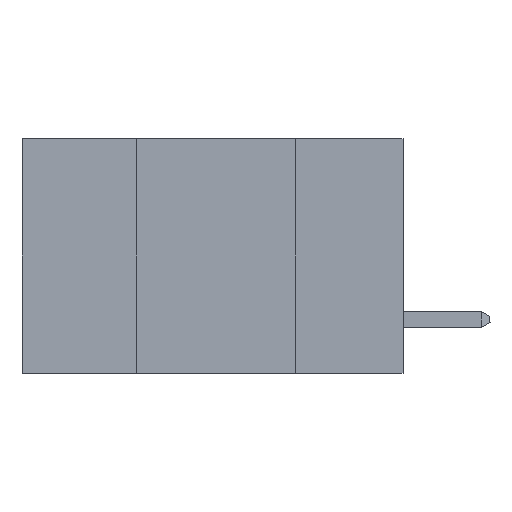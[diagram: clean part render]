
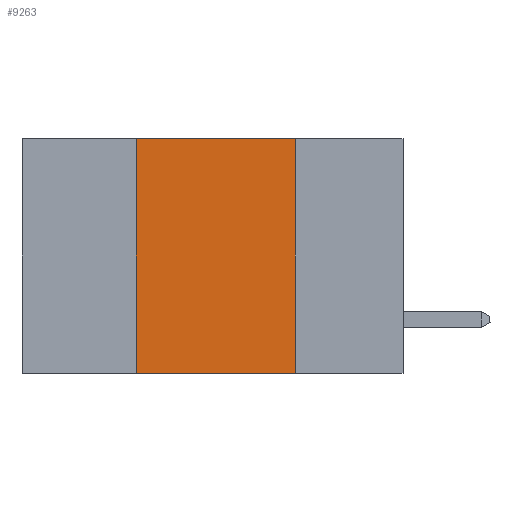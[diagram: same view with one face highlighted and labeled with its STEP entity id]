
A CAD part, left-side view. The second image highlights one B-rep face of the part: STEP entity #9263.
In plain terms, the highlighted planar face has unit normal (-1, 0, 0).
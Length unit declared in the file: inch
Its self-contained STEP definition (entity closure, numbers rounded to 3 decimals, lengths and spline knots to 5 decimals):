
#271 = CARTESIAN_POINT ( 'NONE',  ( 0., 0.6, 0. ) ) ;
#1824 = LINE ( 'NONE', #16335, #13165 ) ;
#4355 = VECTOR ( 'NONE', #14549, 39.37008 ) ;
#4760 = LINE ( 'NONE', #27559, #16158 ) ;
#5156 = ORIENTED_EDGE ( 'NONE', *, *, #15956, .T. ) ;
#5403 = VECTOR ( 'NONE', #34774, 39.37008 ) ;
#5740 = VERTEX_POINT ( 'NONE', #26578 ) ;
#5781 = AXIS2_PLACEMENT_3D ( 'NONE', #271, #24262, #10717 ) ;
#7531 = ORIENTED_EDGE ( 'NONE', *, *, #24913, .F. ) ;
#7590 = ORIENTED_EDGE ( 'NONE', *, *, #16177, .F. ) ;
#8213 = PLANE ( 'NONE',  #5781 ) ;
#8953 = VERTEX_POINT ( 'NONE', #31335 ) ;
#9263 = ADVANCED_FACE ( 'NONE', ( #16354 ), #8213, .F. ) ;
#9565 = CARTESIAN_POINT ( 'NONE',  ( 0., 0.6, -0.37 ) ) ;
#10717 = DIRECTION ( 'NONE',  ( 0., 0., -1. ) ) ;
#10857 = LINE ( 'NONE', #21396, #5403 ) ;
#11183 = ORIENTED_EDGE ( 'NONE', *, *, #21910, .F. ) ;
#13165 = VECTOR ( 'NONE', #16097, 39.37008 ) ;
#14549 = DIRECTION ( 'NONE',  ( 0., -1., 0. ) ) ;
#15956 = EDGE_CURVE ( 'NONE', #22568, #26267, #26698, .T. ) ;
#16097 = DIRECTION ( 'NONE',  ( 0., 0., 1. ) ) ;
#16158 = VECTOR ( 'NONE', #24945, 39.37008 ) ;
#16177 = EDGE_CURVE ( 'NONE', #22568, #5740, #1824, .T. ) ;
#16335 = CARTESIAN_POINT ( 'NONE',  ( 0., 0.42, 0. ) ) ;
#16354 = FACE_OUTER_BOUND ( 'NONE', #21953, .T. ) ;
#17257 = CARTESIAN_POINT ( 'NONE',  ( 0., 0.42, -0.37 ) ) ;
#21396 = CARTESIAN_POINT ( 'NONE',  ( 0., 0.6, 0. ) ) ;
#21910 = EDGE_CURVE ( 'NONE', #5740, #8953, #10857, .T. ) ;
#21953 = EDGE_LOOP ( 'NONE', ( #7531, #11183, #7590, #5156 ) ) ;
#22568 = VERTEX_POINT ( 'NONE', #17257 ) ;
#23654 = CARTESIAN_POINT ( 'NONE',  ( 0., 0.17, -0.37 ) ) ;
#24262 = DIRECTION ( 'NONE',  ( 1., 0., 0. ) ) ;
#24913 = EDGE_CURVE ( 'NONE', #8953, #26267, #4760, .T. ) ;
#24945 = DIRECTION ( 'NONE',  ( 0., 0., -1. ) ) ;
#26267 = VERTEX_POINT ( 'NONE', #23654 ) ;
#26578 = CARTESIAN_POINT ( 'NONE',  ( 0., 0.42, 0. ) ) ;
#26698 = LINE ( 'NONE', #9565, #4355 ) ;
#27559 = CARTESIAN_POINT ( 'NONE',  ( 0., 0.17, 0. ) ) ;
#31335 = CARTESIAN_POINT ( 'NONE',  ( 0., 0.17, 0. ) ) ;
#34774 = DIRECTION ( 'NONE',  ( 0., -1., 0. ) ) ;
